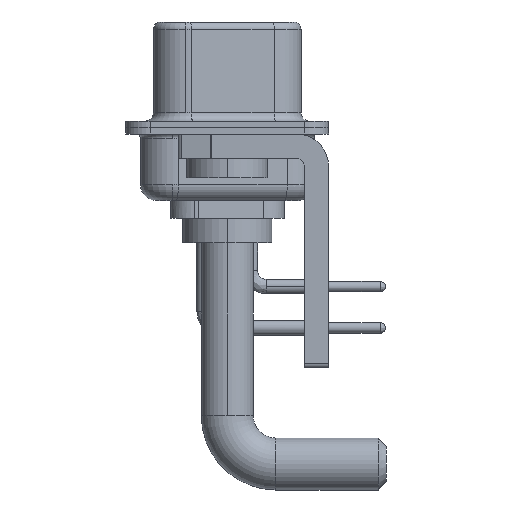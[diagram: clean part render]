
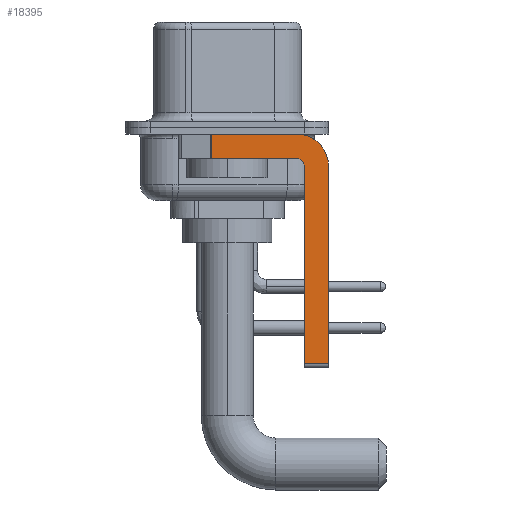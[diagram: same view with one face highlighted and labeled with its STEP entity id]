
A CAD part, left-side view. The second image highlights one B-rep face of the part: STEP entity #18395.
In plain terms, the highlighted planar face has unit normal (-1, 0, 0).
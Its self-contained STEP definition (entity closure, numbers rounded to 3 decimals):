
#79 = CARTESIAN_POINT ( 'NONE',  ( -2.9, -4.25, -1.9 ) ) ;
#215 = CARTESIAN_POINT ( 'NONE',  ( -2.9, -4.25, -14.55 ) ) ;
#610 = VECTOR ( 'NONE', #12245, 1000. ) ;
#1240 = CIRCLE ( 'NONE', #2081, 0.5 ) ;
#1773 = AXIS2_PLACEMENT_3D ( 'NONE', #13506, #11686, #19585 ) ;
#2081 = AXIS2_PLACEMENT_3D ( 'NONE', #13615, #2317, #17072 ) ;
#2317 = DIRECTION ( 'NONE',  ( -1., 0., 0. ) ) ;
#2922 = EDGE_CURVE ( 'NONE', #5936, #13002, #1240, .T. ) ;
#3002 = CARTESIAN_POINT ( 'NONE',  ( -2.9, -4.25, -2.4 ) ) ;
#3418 = VECTOR ( 'NONE', #5364, 1000. ) ;
#4344 = CARTESIAN_POINT ( 'NONE',  ( -2.9, -4.75, -14.55 ) ) ;
#4665 = EDGE_CURVE ( 'NONE', #24502, #5936, #19435, .T. ) ;
#4713 = EDGE_CURVE ( 'NONE', #15088, #12658, #13358, .T. ) ;
#5298 = DIRECTION ( 'NONE',  ( 0., 0., 1. ) ) ;
#5364 = DIRECTION ( 'NONE',  ( 0., 1., 0. ) ) ;
#5418 = AXIS2_PLACEMENT_3D ( 'NONE', #3002, #16523, #22485 ) ;
#5582 = PLANE ( 'NONE',  #1773 ) ;
#5936 = VERTEX_POINT ( 'NONE', #21274 ) ;
#6078 = ORIENTED_EDGE ( 'NONE', *, *, #23383, .F. ) ;
#7251 = CARTESIAN_POINT ( 'NONE',  ( -2.9, -4.75, -14.8 ) ) ;
#7950 = VECTOR ( 'NONE', #5298, 1000. ) ;
#8008 = ORIENTED_EDGE ( 'NONE', *, *, #2922, .F. ) ;
#8349 = VECTOR ( 'NONE', #12613, 1000. ) ;
#8589 = ORIENTED_EDGE ( 'NONE', *, *, #9952, .T. ) ;
#8995 = VERTEX_POINT ( 'NONE', #18079 ) ;
#9847 = CARTESIAN_POINT ( 'NONE',  ( -2.9, -6.25, -14.55 ) ) ;
#9952 = EDGE_CURVE ( 'NONE', #11250, #23323, #15885, .T. ) ;
#10021 = CARTESIAN_POINT ( 'NONE',  ( -2.9, 0.978, -1.9 ) ) ;
#10098 = DIRECTION ( 'NONE',  ( 0., 0., -1. ) ) ;
#11250 = VERTEX_POINT ( 'NONE', #21734 ) ;
#11529 = ORIENTED_EDGE ( 'NONE', *, *, #4665, .F. ) ;
#11686 = DIRECTION ( 'NONE',  ( 1., 0., 0. ) ) ;
#11860 = ORIENTED_EDGE ( 'NONE', *, *, #21821, .F. ) ;
#11912 = DIRECTION ( 'NONE',  ( 0., -1., 0. ) ) ;
#12245 = DIRECTION ( 'NONE',  ( 0., 0., -1. ) ) ;
#12613 = DIRECTION ( 'NONE',  ( 0., -1., 0. ) ) ;
#12658 = VERTEX_POINT ( 'NONE', #9847 ) ;
#13002 = VERTEX_POINT ( 'NONE', #79 ) ;
#13358 = LINE ( 'NONE', #17381, #18734 ) ;
#13506 = CARTESIAN_POINT ( 'NONE',  ( -2.9, -4.25, -2.4 ) ) ;
#13615 = CARTESIAN_POINT ( 'NONE',  ( -2.9, -4.25, -2.4 ) ) ;
#14012 = CARTESIAN_POINT ( 'NONE',  ( -2.9, -6.25, -2.4 ) ) ;
#14246 = EDGE_CURVE ( 'NONE', #24502, #12658, #23584, .T. ) ;
#15088 = VERTEX_POINT ( 'NONE', #14012 ) ;
#15885 = LINE ( 'NONE', #10021, #610 ) ;
#16523 = DIRECTION ( 'NONE',  ( 1., 0., 0. ) ) ;
#16625 = CIRCLE ( 'NONE', #5418, 2. ) ;
#16803 = EDGE_CURVE ( 'NONE', #11250, #8995, #18814, .T. ) ;
#16922 = ORIENTED_EDGE ( 'NONE', *, *, #4713, .F. ) ;
#17072 = DIRECTION ( 'NONE',  ( 0., 0., 1. ) ) ;
#17381 = CARTESIAN_POINT ( 'NONE',  ( -2.9, -6.25, -2.4 ) ) ;
#17959 = ORIENTED_EDGE ( 'NONE', *, *, #14246, .T. ) ;
#18079 = CARTESIAN_POINT ( 'NONE',  ( -2.9, -4.25, -0.4 ) ) ;
#18395 = ADVANCED_FACE ( 'NONE', ( #25077 ), #5582, .F. ) ;
#18734 = VECTOR ( 'NONE', #10098, 1000. ) ;
#18814 = LINE ( 'NONE', #22852, #8349 ) ;
#19435 = LINE ( 'NONE', #7251, #7950 ) ;
#19585 = DIRECTION ( 'NONE',  ( 0., 0., -1. ) ) ;
#20622 = ORIENTED_EDGE ( 'NONE', *, *, #16803, .F. ) ;
#21274 = CARTESIAN_POINT ( 'NONE',  ( -2.9, -4.75, -2.4 ) ) ;
#21734 = CARTESIAN_POINT ( 'NONE',  ( -2.9, 0.978, -0.4 ) ) ;
#21821 = EDGE_CURVE ( 'NONE', #8995, #15088, #16625, .T. ) ;
#22418 = VECTOR ( 'NONE', #11912, 1000. ) ;
#22485 = DIRECTION ( 'NONE',  ( 0., 0., -1. ) ) ;
#22644 = CARTESIAN_POINT ( 'NONE',  ( -2.9, 0.978, -1.9 ) ) ;
#22852 = CARTESIAN_POINT ( 'NONE',  ( -2.9, 3., -0.4 ) ) ;
#23289 = LINE ( 'NONE', #24989, #3418 ) ;
#23323 = VERTEX_POINT ( 'NONE', #22644 ) ;
#23383 = EDGE_CURVE ( 'NONE', #13002, #23323, #23289, .T. ) ;
#23584 = LINE ( 'NONE', #215, #22418 ) ;
#24048 = EDGE_LOOP ( 'NONE', ( #20622, #8589, #6078, #8008, #11529, #17959, #16922, #11860 ) ) ;
#24502 = VERTEX_POINT ( 'NONE', #4344 ) ;
#24989 = CARTESIAN_POINT ( 'NONE',  ( -2.9, -4.25, -1.9 ) ) ;
#25077 = FACE_OUTER_BOUND ( 'NONE', #24048, .T. ) ;
